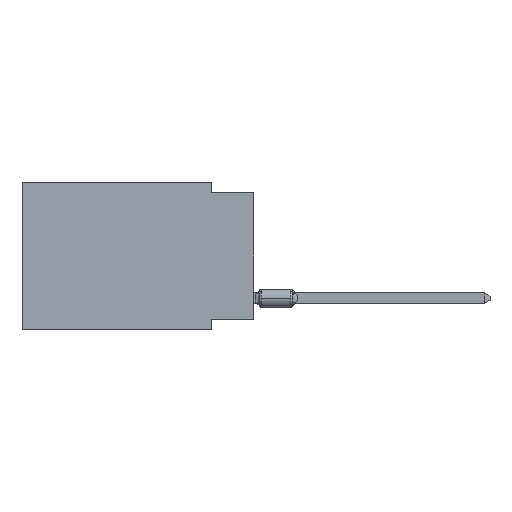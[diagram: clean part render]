
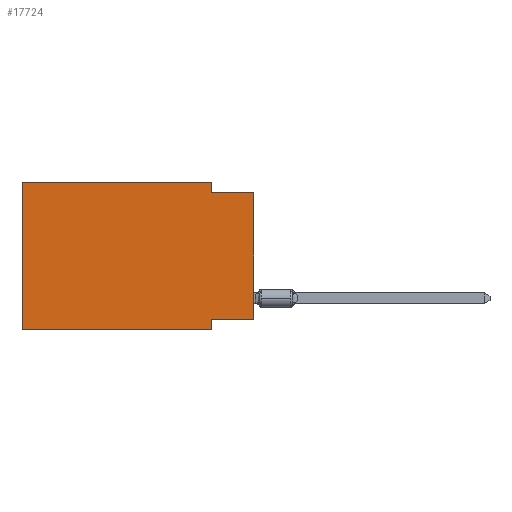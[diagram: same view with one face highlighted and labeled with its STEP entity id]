
A CAD part, left-side view. The second image highlights one B-rep face of the part: STEP entity #17724.
In plain terms, the highlighted planar face has unit normal (-1, 0, 0).
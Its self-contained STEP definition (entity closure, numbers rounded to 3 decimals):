
#342 = ORIENTED_EDGE ( 'NONE', *, *, #15616, .F. ) ;
#1206 = CARTESIAN_POINT ( 'NONE',  ( 0., 13.97, -8.89 ) ) ;
#1219 = CARTESIAN_POINT ( 'NONE',  ( 0., 0., 0. ) ) ;
#1739 = CARTESIAN_POINT ( 'NONE',  ( 0., 2.54, -0.635 ) ) ;
#3417 = CARTESIAN_POINT ( 'NONE',  ( 0., 2.54, -8.89 ) ) ;
#3460 = CARTESIAN_POINT ( 'NONE',  ( 0., 13.97, -8.89 ) ) ;
#3953 = LINE ( 'NONE', #20513, #15839 ) ;
#4598 = VECTOR ( 'NONE', #28038, 1000. ) ;
#5110 = PLANE ( 'NONE',  #20701 ) ;
#5492 = LINE ( 'NONE', #24619, #26030 ) ;
#6529 = CARTESIAN_POINT ( 'NONE',  ( 0., 13.97, 0. ) ) ;
#6947 = CARTESIAN_POINT ( 'NONE',  ( 0., 2.54, 0. ) ) ;
#7569 = VECTOR ( 'NONE', #28927, 1000. ) ;
#9447 = VERTEX_POINT ( 'NONE', #13148 ) ;
#10158 = EDGE_CURVE ( 'NONE', #9447, #11348, #11558, .T. ) ;
#10199 = EDGE_LOOP ( 'NONE', ( #16708, #17326, #17376, #342, #18297, #17991, #27498, #18472 ) ) ;
#10886 = LINE ( 'NONE', #28083, #19002 ) ;
#10905 = CARTESIAN_POINT ( 'NONE',  ( 0., 2.54, -8.255 ) ) ;
#11348 = VERTEX_POINT ( 'NONE', #1739 ) ;
#11558 = LINE ( 'NONE', #6947, #7569 ) ;
#12332 = DIRECTION ( 'NONE',  ( 0., -1., 0. ) ) ;
#12344 = EDGE_CURVE ( 'NONE', #11348, #15956, #3953, .T. ) ;
#13008 = LINE ( 'NONE', #3460, #21922 ) ;
#13117 = DIRECTION ( 'NONE',  ( 0., 0., -1. ) ) ;
#13148 = CARTESIAN_POINT ( 'NONE',  ( 0., 2.54, 0. ) ) ;
#13628 = EDGE_CURVE ( 'NONE', #15812, #16047, #20869, .T. ) ;
#13647 = DIRECTION ( 'NONE',  ( 0., -1., 0. ) ) ;
#13880 = CARTESIAN_POINT ( 'NONE',  ( 0., 2.54, -8.89 ) ) ;
#13886 = VECTOR ( 'NONE', #20462, 1000. ) ;
#15287 = DIRECTION ( 'NONE',  ( 1., 0., 0. ) ) ;
#15383 = EDGE_CURVE ( 'NONE', #15812, #28498, #13008, .T. ) ;
#15616 = EDGE_CURVE ( 'NONE', #16047, #9447, #5492, .T. ) ;
#15812 = VERTEX_POINT ( 'NONE', #1206 ) ;
#15839 = VECTOR ( 'NONE', #13647, 1000. ) ;
#15956 = VERTEX_POINT ( 'NONE', #23634 ) ;
#16047 = VERTEX_POINT ( 'NONE', #17236 ) ;
#16708 = ORIENTED_EDGE ( 'NONE', *, *, #29202, .T. ) ;
#17236 = CARTESIAN_POINT ( 'NONE',  ( 0., 13.97, 0. ) ) ;
#17326 = ORIENTED_EDGE ( 'NONE', *, *, #12344, .F. ) ;
#17376 = ORIENTED_EDGE ( 'NONE', *, *, #10158, .F. ) ;
#17724 = ADVANCED_FACE ( 'NONE', ( #22293 ), #5110, .F. ) ;
#17991 = ORIENTED_EDGE ( 'NONE', *, *, #15383, .T. ) ;
#18297 = ORIENTED_EDGE ( 'NONE', *, *, #13628, .F. ) ;
#18472 = ORIENTED_EDGE ( 'NONE', *, *, #31294, .F. ) ;
#19002 = VECTOR ( 'NONE', #30320, 1000. ) ;
#19954 = CARTESIAN_POINT ( 'NONE',  ( 0., 0., -8.255 ) ) ;
#20462 = DIRECTION ( 'NONE',  ( 0., 0., 1. ) ) ;
#20513 = CARTESIAN_POINT ( 'NONE',  ( 0., 0., -0.635 ) ) ;
#20701 = AXIS2_PLACEMENT_3D ( 'NONE', #24548, #15287, #25176 ) ;
#20869 = LINE ( 'NONE', #6529, #4598 ) ;
#21922 = VECTOR ( 'NONE', #23341, 1000. ) ;
#22293 = FACE_OUTER_BOUND ( 'NONE', #10199, .T. ) ;
#22542 = LINE ( 'NONE', #1219, #13886 ) ;
#23341 = DIRECTION ( 'NONE',  ( 0., -1., 0. ) ) ;
#23634 = CARTESIAN_POINT ( 'NONE',  ( 0., 0., -0.635 ) ) ;
#24548 = CARTESIAN_POINT ( 'NONE',  ( 0., 13.97, 0. ) ) ;
#24619 = CARTESIAN_POINT ( 'NONE',  ( 0., 13.97, 0. ) ) ;
#25176 = DIRECTION ( 'NONE',  ( 0., 0., -1. ) ) ;
#25230 = LINE ( 'NONE', #3417, #25627 ) ;
#25555 = VERTEX_POINT ( 'NONE', #19954 ) ;
#25627 = VECTOR ( 'NONE', #13117, 1000. ) ;
#26030 = VECTOR ( 'NONE', #12332, 1000. ) ;
#27498 = ORIENTED_EDGE ( 'NONE', *, *, #30098, .F. ) ;
#28038 = DIRECTION ( 'NONE',  ( 0., 0., 1. ) ) ;
#28083 = CARTESIAN_POINT ( 'NONE',  ( 0., 0., -8.255 ) ) ;
#28498 = VERTEX_POINT ( 'NONE', #13880 ) ;
#28927 = DIRECTION ( 'NONE',  ( 0., 0., -1. ) ) ;
#29140 = VERTEX_POINT ( 'NONE', #10905 ) ;
#29202 = EDGE_CURVE ( 'NONE', #25555, #15956, #22542, .T. ) ;
#30098 = EDGE_CURVE ( 'NONE', #29140, #28498, #25230, .T. ) ;
#30320 = DIRECTION ( 'NONE',  ( 0., 1., 0. ) ) ;
#31294 = EDGE_CURVE ( 'NONE', #25555, #29140, #10886, .T. ) ;
